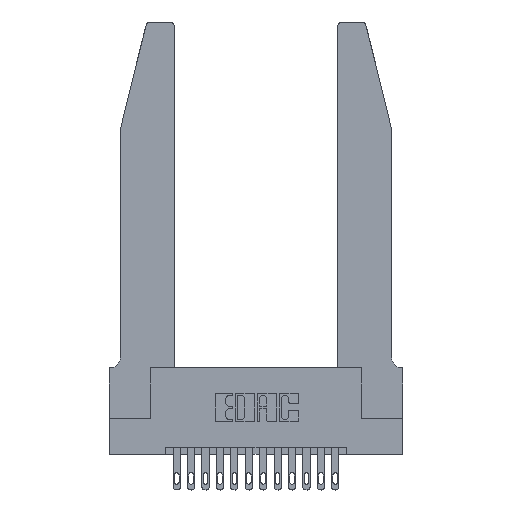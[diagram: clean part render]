
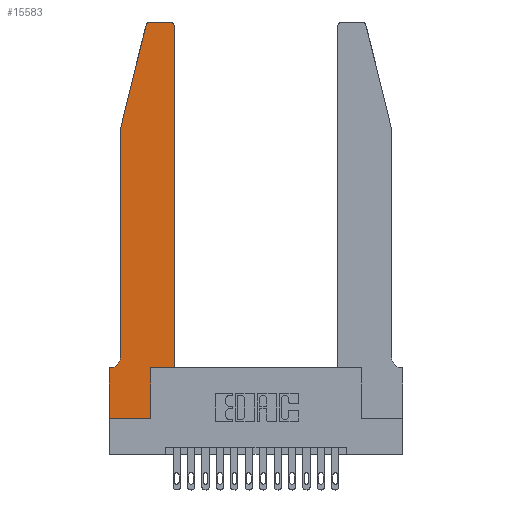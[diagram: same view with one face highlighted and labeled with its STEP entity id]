
A CAD part, top view. The second image highlights one B-rep face of the part: STEP entity #15583.
In plain terms, the highlighted planar face has unit normal (0, 0, 1).
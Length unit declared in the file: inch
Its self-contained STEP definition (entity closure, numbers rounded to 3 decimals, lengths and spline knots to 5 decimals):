
#154 = VERTEX_POINT ( 'NONE', #15360 ) ;
#180 = DIRECTION ( 'NONE',  ( -1., 0., 0. ) ) ;
#214 = DIRECTION ( 'NONE',  ( 0., 1., 0. ) ) ;
#277 = CARTESIAN_POINT ( 'NONE',  ( 0.4205, 2.72, 0.37 ) ) ;
#287 = VERTEX_POINT ( 'NONE', #14382 ) ;
#341 = ORIENTED_EDGE ( 'NONE', *, *, #13249, .T. ) ;
#429 = EDGE_CURVE ( 'NONE', #17630, #6670, #4827, .T. ) ;
#501 = DIRECTION ( 'NONE',  ( 0., -1., 0. ) ) ;
#633 = ORIENTED_EDGE ( 'NONE', *, *, #8999, .T. ) ;
#828 = CARTESIAN_POINT ( 'NONE',  ( 0.4205, 2.75, 0.37 ) ) ;
#970 = VERTEX_POINT ( 'NONE', #11132 ) ;
#1136 = CARTESIAN_POINT ( 'NONE',  ( 0.4505, 0.35, 0.37 ) ) ;
#1255 = LINE ( 'NONE', #1718, #14591 ) ;
#1575 = EDGE_CURVE ( 'NONE', #10466, #154, #12365, .T. ) ;
#1644 = DIRECTION ( 'NONE',  ( 1., 0., 0. ) ) ;
#1718 = CARTESIAN_POINT ( 'NONE',  ( 0., 0., 0.37 ) ) ;
#1784 = LINE ( 'NONE', #15794, #13382 ) ;
#1840 = ORIENTED_EDGE ( 'NONE', *, *, #5937, .T. ) ;
#2361 = VERTEX_POINT ( 'NONE', #12216 ) ;
#2551 = LINE ( 'NONE', #13544, #15004 ) ;
#2913 = ORIENTED_EDGE ( 'NONE', *, *, #6798, .T. ) ;
#2924 = VERTEX_POINT ( 'NONE', #16178 ) ;
#3162 = LINE ( 'NONE', #5382, #6845 ) ;
#3922 = AXIS2_PLACEMENT_3D ( 'NONE', #8310, #13808, #8370 ) ;
#4027 = AXIS2_PLACEMENT_3D ( 'NONE', #5792, #16954, #180 ) ;
#4096 = EDGE_CURVE ( 'NONE', #2924, #13615, #11697, .T. ) ;
#4165 = PLANE ( 'NONE',  #10123 ) ;
#4327 = CARTESIAN_POINT ( 'NONE',  ( 0.4505, 0.35, 0.37 ) ) ;
#4476 = LINE ( 'NONE', #7473, #15635 ) ;
#4523 = VERTEX_POINT ( 'NONE', #1136 ) ;
#4827 = LINE ( 'NONE', #14688, #5272 ) ;
#4831 = ORIENTED_EDGE ( 'NONE', *, *, #5171, .T. ) ;
#4910 = CARTESIAN_POINT ( 'NONE',  ( 0., 0.35, 0.37 ) ) ;
#5049 = CARTESIAN_POINT ( 'NONE',  ( 0.0055, 0.35, 0.37 ) ) ;
#5122 = EDGE_CURVE ( 'NONE', #287, #970, #1255, .T. ) ;
#5159 = DIRECTION ( 'NONE',  ( -1., 0., 0. ) ) ;
#5171 = EDGE_CURVE ( 'NONE', #154, #17630, #17219, .T. ) ;
#5272 = VECTOR ( 'NONE', #13403, 39.37008 ) ;
#5382 = CARTESIAN_POINT ( 'NONE',  ( 0.4505, 0.35, 0.37 ) ) ;
#5383 = CARTESIAN_POINT ( 'NONE',  ( 0.0755, 2., 0.37 ) ) ;
#5494 = EDGE_CURVE ( 'NONE', #5702, #2361, #15890, .T. ) ;
#5702 = VERTEX_POINT ( 'NONE', #12998 ) ;
#5792 = CARTESIAN_POINT ( 'NONE',  ( 0.0055, 0.42, 0.37 ) ) ;
#5937 = EDGE_CURVE ( 'NONE', #13615, #5702, #2551, .T. ) ;
#6361 = EDGE_CURVE ( 'NONE', #6670, #287, #4476, .T. ) ;
#6383 = ORIENTED_EDGE ( 'NONE', *, *, #1575, .T. ) ;
#6670 = VERTEX_POINT ( 'NONE', #4910 ) ;
#6798 = EDGE_CURVE ( 'NONE', #2361, #10466, #16505, .T. ) ;
#6845 = VECTOR ( 'NONE', #6956, 39.37008 ) ;
#6956 = DIRECTION ( 'NONE',  ( 1., 0., 0. ) ) ;
#7473 = CARTESIAN_POINT ( 'NONE',  ( 0., 0., 0.37 ) ) ;
#7484 = EDGE_CURVE ( 'NONE', #10832, #4523, #3162, .T. ) ;
#7518 = LINE ( 'NONE', #4327, #8188 ) ;
#8188 = VECTOR ( 'NONE', #214, 39.37008 ) ;
#8310 = CARTESIAN_POINT ( 'NONE',  ( 0.284, 2.72, 0.37 ) ) ;
#8370 = DIRECTION ( 'NONE',  ( 1., 0., 0. ) ) ;
#8999 = EDGE_CURVE ( 'NONE', #970, #10832, #1784, .T. ) ;
#9172 = AXIS2_PLACEMENT_3D ( 'NONE', #277, #14405, #1644 ) ;
#9241 = VECTOR ( 'NONE', #9499, 39.37008 ) ;
#9292 = ORIENTED_EDGE ( 'NONE', *, *, #7484, .T. ) ;
#9499 = DIRECTION ( 'NONE',  ( 0., -1., 0. ) ) ;
#9951 = ORIENTED_EDGE ( 'NONE', *, *, #5494, .T. ) ;
#10084 = DIRECTION ( 'NONE',  ( 1., 0., 0. ) ) ;
#10123 = AXIS2_PLACEMENT_3D ( 'NONE', #18000, #11062, #15211 ) ;
#10466 = VERTEX_POINT ( 'NONE', #18098 ) ;
#10832 = VERTEX_POINT ( 'NONE', #12060 ) ;
#10962 = FACE_OUTER_BOUND ( 'NONE', #17905, .T. ) ;
#11038 = CARTESIAN_POINT ( 'NONE',  ( 0.0755, 2., 0.37 ) ) ;
#11062 = DIRECTION ( 'NONE',  ( 0., 0., 1. ) ) ;
#11132 = CARTESIAN_POINT ( 'NONE',  ( 0.2865, 0., 0.37 ) ) ;
#11457 = VECTOR ( 'NONE', #12438, 39.37008 ) ;
#11697 = CIRCLE ( 'NONE', #9172, 0.03 ) ;
#12060 = CARTESIAN_POINT ( 'NONE',  ( 0.2865, 0.35, 0.37 ) ) ;
#12216 = CARTESIAN_POINT ( 'NONE',  ( 0.25487, 2.72718, 0.37 ) ) ;
#12365 = LINE ( 'NONE', #5383, #9241 ) ;
#12438 = DIRECTION ( 'NONE',  ( -0.239, -0.971, 0. ) ) ;
#12998 = CARTESIAN_POINT ( 'NONE',  ( 0.284, 2.75, 0.37 ) ) ;
#13249 = EDGE_CURVE ( 'NONE', #4523, #2924, #7518, .T. ) ;
#13303 = ORIENTED_EDGE ( 'NONE', *, *, #6361, .T. ) ;
#13382 = VECTOR ( 'NONE', #15603, 39.37008 ) ;
#13403 = DIRECTION ( 'NONE',  ( -1., 0., 0. ) ) ;
#13544 = CARTESIAN_POINT ( 'NONE',  ( 0.2605, 2.75, 0.37 ) ) ;
#13615 = VERTEX_POINT ( 'NONE', #828 ) ;
#13808 = DIRECTION ( 'NONE',  ( 0., 0., 1. ) ) ;
#14258 = ORIENTED_EDGE ( 'NONE', *, *, #5122, .T. ) ;
#14382 = CARTESIAN_POINT ( 'NONE',  ( 0., 0., 0.37 ) ) ;
#14405 = DIRECTION ( 'NONE',  ( 0., 0., 1. ) ) ;
#14590 = ORIENTED_EDGE ( 'NONE', *, *, #4096, .T. ) ;
#14591 = VECTOR ( 'NONE', #10084, 39.37008 ) ;
#14688 = CARTESIAN_POINT ( 'NONE',  ( 0.0755, 0.35, 0.37 ) ) ;
#15004 = VECTOR ( 'NONE', #5159, 39.37008 ) ;
#15211 = DIRECTION ( 'NONE',  ( 1., 0., 0. ) ) ;
#15360 = CARTESIAN_POINT ( 'NONE',  ( 0.0755, 0.42, 0.37 ) ) ;
#15583 = ADVANCED_FACE ( 'NONE', ( #10962 ), #4165, .T. ) ;
#15603 = DIRECTION ( 'NONE',  ( 0., 1., 0. ) ) ;
#15635 = VECTOR ( 'NONE', #501, 39.37008 ) ;
#15794 = CARTESIAN_POINT ( 'NONE',  ( 0.2865, 0.35, 0.37 ) ) ;
#15890 = CIRCLE ( 'NONE', #3922, 0.03 ) ;
#16151 = ORIENTED_EDGE ( 'NONE', *, *, #429, .T. ) ;
#16178 = CARTESIAN_POINT ( 'NONE',  ( 0.4505, 2.72, 0.37 ) ) ;
#16505 = LINE ( 'NONE', #11038, #11457 ) ;
#16954 = DIRECTION ( 'NONE',  ( 0., 0., -1. ) ) ;
#17219 = CIRCLE ( 'NONE', #4027, 0.07 ) ;
#17630 = VERTEX_POINT ( 'NONE', #5049 ) ;
#17905 = EDGE_LOOP ( 'NONE', ( #1840, #9951, #2913, #6383, #4831, #16151, #13303, #14258, #633, #9292, #341, #14590 ) ) ;
#18000 = CARTESIAN_POINT ( 'NONE',  ( 0., 0.35, 0.37 ) ) ;
#18098 = CARTESIAN_POINT ( 'NONE',  ( 0.0755, 2., 0.37 ) ) ;
